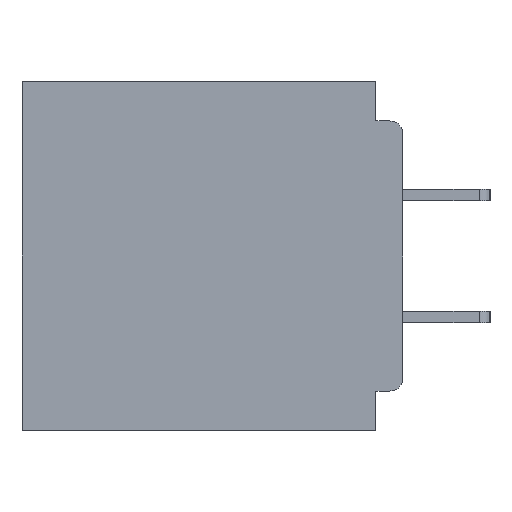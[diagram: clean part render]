
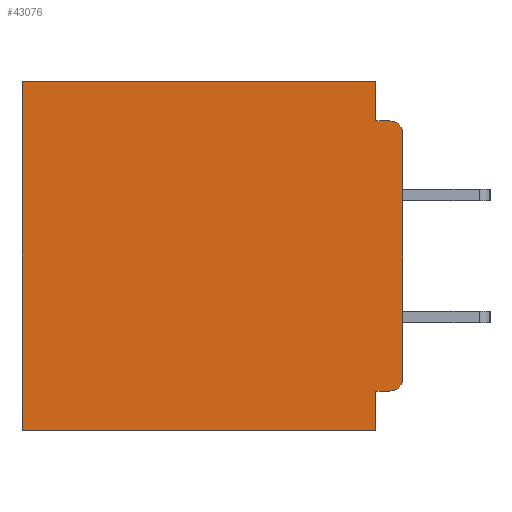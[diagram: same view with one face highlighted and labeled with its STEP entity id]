
A CAD part, left-side view. The second image highlights one B-rep face of the part: STEP entity #43076.
In plain terms, the highlighted planar face has unit normal (-1, 0, 0).
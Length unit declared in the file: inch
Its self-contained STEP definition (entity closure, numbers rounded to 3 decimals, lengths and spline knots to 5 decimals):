
#27 = FACE_OUTER_BOUND ( 'NONE', #37024, .T. ) ;
#1409 = LINE ( 'NONE', #19746, #35656 ) ;
#2090 = VECTOR ( 'NONE', #3413, 39.37008 ) ;
#2811 = VECTOR ( 'NONE', #54764, 39.37008 ) ;
#3396 = ORIENTED_EDGE ( 'NONE', *, *, #20547, .F. ) ;
#3413 = DIRECTION ( 'NONE',  ( 0., 0., -1. ) ) ;
#5746 = LINE ( 'NONE', #50112, #2811 ) ;
#6878 = CARTESIAN_POINT ( 'NONE',  ( 0.3, 0.015, -0.34 ) ) ;
#6901 = DIRECTION ( 'NONE',  ( 0., 1., 0. ) ) ;
#7627 = EDGE_CURVE ( 'NONE', #52373, #45547, #9784, .T. ) ;
#7858 = VERTEX_POINT ( 'NONE', #47734 ) ;
#8475 = AXIS2_PLACEMENT_3D ( 'NONE', #39303, #11424, #43959 ) ;
#8657 = ORIENTED_EDGE ( 'NONE', *, *, #15931, .F. ) ;
#9784 = CIRCLE ( 'NONE', #40073, 0.015 ) ;
#10540 = DIRECTION ( 'NONE',  ( 0., 1., 0. ) ) ;
#11424 = DIRECTION ( 'NONE',  ( 1., 0., 0. ) ) ;
#11568 = DIRECTION ( 'NONE',  ( 0., 0., -1. ) ) ;
#12686 = VERTEX_POINT ( 'NONE', #53371 ) ;
#13304 = LINE ( 'NONE', #44132, #35142 ) ;
#13615 = DIRECTION ( 'NONE',  ( 0., 0., -1. ) ) ;
#13657 = VERTEX_POINT ( 'NONE', #50837 ) ;
#13829 = CARTESIAN_POINT ( 'NONE',  ( 0.3, 0.015, -0.06 ) ) ;
#13868 = EDGE_CURVE ( 'NONE', #18333, #35557, #49489, .T. ) ;
#14124 = CARTESIAN_POINT ( 'NONE',  ( 0.3, 0., -0.34 ) ) ;
#14674 = EDGE_CURVE ( 'NONE', #13657, #45547, #5746, .T. ) ;
#15903 = PLANE ( 'NONE',  #8475 ) ;
#15931 = EDGE_CURVE ( 'NONE', #18333, #7858, #1409, .T. ) ;
#15979 = VECTOR ( 'NONE', #22876, 39.37008 ) ;
#16234 = EDGE_CURVE ( 'NONE', #32437, #21850, #45760, .T. ) ;
#17981 = CARTESIAN_POINT ( 'NONE',  ( 0.3, 0.015, -0.355 ) ) ;
#17994 = CARTESIAN_POINT ( 'NONE',  ( 0.3, 0.031, 0. ) ) ;
#18303 = CARTESIAN_POINT ( 'NONE',  ( 0.3, 0.031, -0.4 ) ) ;
#18333 = VERTEX_POINT ( 'NONE', #17981 ) ;
#18527 = DIRECTION ( 'NONE',  ( 0., 0., -1. ) ) ;
#18894 = AXIS2_PLACEMENT_3D ( 'NONE', #6878, #39463, #11568 ) ;
#19298 = ORIENTED_EDGE ( 'NONE', *, *, #7627, .T. ) ;
#19746 = CARTESIAN_POINT ( 'NONE',  ( 0.3, 0., -0.355 ) ) ;
#19919 = CARTESIAN_POINT ( 'NONE',  ( 0.3, 0., -0.4 ) ) ;
#20547 = EDGE_CURVE ( 'NONE', #53876, #21850, #13304, .T. ) ;
#21485 = ORIENTED_EDGE ( 'NONE', *, *, #14674, .F. ) ;
#21850 = VERTEX_POINT ( 'NONE', #57778 ) ;
#22876 = DIRECTION ( 'NONE',  ( 0., 0., -1. ) ) ;
#22918 = LINE ( 'NONE', #19919, #47602 ) ;
#26526 = VECTOR ( 'NONE', #34987, 39.37008 ) ;
#29159 = EDGE_CURVE ( 'NONE', #7858, #53876, #47591, .T. ) ;
#31744 = EDGE_CURVE ( 'NONE', #12686, #13657, #42167, .T. ) ;
#32437 = VERTEX_POINT ( 'NONE', #32572 ) ;
#32572 = CARTESIAN_POINT ( 'NONE',  ( 0.3, 0.437, 0. ) ) ;
#34985 = CARTESIAN_POINT ( 'NONE',  ( 0.3, 0.015, -0.045 ) ) ;
#34987 = DIRECTION ( 'NONE',  ( 0., 1., 0. ) ) ;
#35142 = VECTOR ( 'NONE', #6901, 39.37008 ) ;
#35557 = VERTEX_POINT ( 'NONE', #14124 ) ;
#35656 = VECTOR ( 'NONE', #10540, 39.37008 ) ;
#35983 = CARTESIAN_POINT ( 'NONE',  ( 0.3, 0.437, -0.4 ) ) ;
#37024 = EDGE_LOOP ( 'NONE', ( #53654, #19298, #21485, #51615, #50186, #53734, #3396, #56078, #8657, #50183 ) ) ;
#37287 = EDGE_CURVE ( 'NONE', #12686, #32437, #51194, .T. ) ;
#39303 = CARTESIAN_POINT ( 'NONE',  ( 0.3, 0., -0.4 ) ) ;
#39463 = DIRECTION ( 'NONE',  ( -1., 0., 0. ) ) ;
#40073 = AXIS2_PLACEMENT_3D ( 'NONE', #13829, #46338, #18527 ) ;
#42167 = LINE ( 'NONE', #17994, #15979 ) ;
#43076 = ADVANCED_FACE ( 'NONE', ( #27 ), #15903, .F. ) ;
#43959 = DIRECTION ( 'NONE',  ( 0., 0., -1. ) ) ;
#44087 = CARTESIAN_POINT ( 'NONE',  ( 0.3, 0., 0. ) ) ;
#44132 = CARTESIAN_POINT ( 'NONE',  ( 0.3, 0., -0.4 ) ) ;
#45547 = VERTEX_POINT ( 'NONE', #34985 ) ;
#45760 = LINE ( 'NONE', #35983, #2090 ) ;
#46338 = DIRECTION ( 'NONE',  ( -1., 0., 0. ) ) ;
#47591 = LINE ( 'NONE', #18303, #58494 ) ;
#47602 = VECTOR ( 'NONE', #52413, 39.37008 ) ;
#47734 = CARTESIAN_POINT ( 'NONE',  ( 0.3, 0.031, -0.355 ) ) ;
#47745 = CARTESIAN_POINT ( 'NONE',  ( 0.3, 0., -0.06 ) ) ;
#49489 = CIRCLE ( 'NONE', #18894, 0.015 ) ;
#49680 = CARTESIAN_POINT ( 'NONE',  ( 0.3, 0.031, -0.4 ) ) ;
#50112 = CARTESIAN_POINT ( 'NONE',  ( 0.3, 0., -0.045 ) ) ;
#50183 = ORIENTED_EDGE ( 'NONE', *, *, #13868, .T. ) ;
#50186 = ORIENTED_EDGE ( 'NONE', *, *, #37287, .T. ) ;
#50837 = CARTESIAN_POINT ( 'NONE',  ( 0.3, 0.031, -0.045 ) ) ;
#51194 = LINE ( 'NONE', #44087, #26526 ) ;
#51615 = ORIENTED_EDGE ( 'NONE', *, *, #31744, .F. ) ;
#52373 = VERTEX_POINT ( 'NONE', #47745 ) ;
#52413 = DIRECTION ( 'NONE',  ( 0., 0., -1. ) ) ;
#53371 = CARTESIAN_POINT ( 'NONE',  ( 0.3, 0.031, 0. ) ) ;
#53654 = ORIENTED_EDGE ( 'NONE', *, *, #54866, .F. ) ;
#53734 = ORIENTED_EDGE ( 'NONE', *, *, #16234, .T. ) ;
#53876 = VERTEX_POINT ( 'NONE', #49680 ) ;
#54764 = DIRECTION ( 'NONE',  ( 0., -1., 0. ) ) ;
#54866 = EDGE_CURVE ( 'NONE', #52373, #35557, #22918, .T. ) ;
#56078 = ORIENTED_EDGE ( 'NONE', *, *, #29159, .F. ) ;
#57778 = CARTESIAN_POINT ( 'NONE',  ( 0.3, 0.437, -0.4 ) ) ;
#58494 = VECTOR ( 'NONE', #13615, 39.37008 ) ;
